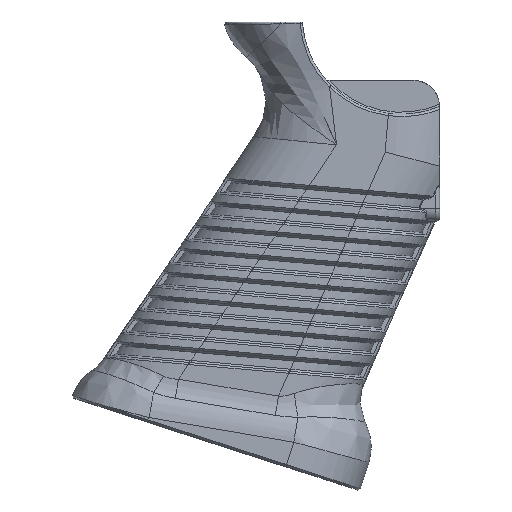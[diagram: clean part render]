
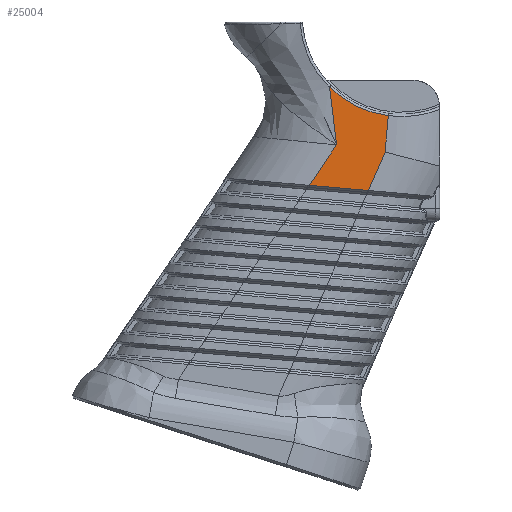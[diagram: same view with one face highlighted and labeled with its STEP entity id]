
A CAD part, top view. The second image highlights one B-rep face of the part: STEP entity #25004.
In plain terms, the highlighted planar face has unit normal (0, 0, 1).
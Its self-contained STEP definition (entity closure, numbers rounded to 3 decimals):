
#43 = DIRECTION ( 'NONE',  ( 0., 0., -1. ) ) ;
#418 = ORIENTED_EDGE ( 'NONE', *, *, #11434, .F. ) ;
#522 = DIRECTION ( 'NONE',  ( 0., 0., 1. ) ) ;
#1419 = VECTOR ( 'NONE', #10478, 1000. ) ;
#3633 = CARTESIAN_POINT ( 'NONE',  ( -142.328, -35.946, 17.501 ) ) ;
#3802 = VECTOR ( 'NONE', #4285, 1000. ) ;
#4087 = LINE ( 'NONE', #6663, #24403 ) ;
#4285 = DIRECTION ( 'NONE',  ( -0.996, 0.087, 0. ) ) ;
#4435 = VERTEX_POINT ( 'NONE', #27079 ) ;
#4528 = VERTEX_POINT ( 'NONE', #9547 ) ;
#5375 = EDGE_CURVE ( 'NONE', #19435, #14059, #4087, .T. ) ;
#5696 = LINE ( 'NONE', #3633, #17031 ) ;
#5759 = EDGE_CURVE ( 'NONE', #14059, #4528, #22493, .T. ) ;
#5824 = CARTESIAN_POINT ( 'NONE',  ( -158.322, -37.684, 17.501 ) ) ;
#6024 = CARTESIAN_POINT ( 'NONE',  ( -159.225, -30.876, 17.501 ) ) ;
#6251 = CARTESIAN_POINT ( 'NONE',  ( -158.847, -33.206, 17.501 ) ) ;
#6663 = CARTESIAN_POINT ( 'NONE',  ( -146.326, -26.223, 17.501 ) ) ;
#7158 = ORIENTED_EDGE ( 'NONE', *, *, #5759, .F. ) ;
#7208 = CARTESIAN_POINT ( 'NONE',  ( -132.232, -35.729, 17.501 ) ) ;
#7649 = FACE_OUTER_BOUND ( 'NONE', #9643, .T. ) ;
#7962 = CARTESIAN_POINT ( 'NONE',  ( -164.336, -52.925, 17.501 ) ) ;
#8347 = CARTESIAN_POINT ( 'NONE',  ( -159.467, -29.661, 17.501 ) ) ;
#9547 = CARTESIAN_POINT ( 'NONE',  ( -159.489, -29.553, 17.501 ) ) ;
#9643 = EDGE_LOOP ( 'NONE', ( #418, #7158, #22928, #22411, #29235, #12573, #22606 ) ) ;
#9734 = CARTESIAN_POINT ( 'NONE',  ( -145.543, -36.362, 17.501 ) ) ;
#9967 = DIRECTION ( 'NONE',  ( -0.559, -0.829, 0. ) ) ;
#10478 = DIRECTION ( 'NONE',  ( -0.996, 0.087, 0. ) ) ;
#10980 = CARTESIAN_POINT ( 'NONE',  ( -158.047, -41.059, 17.501 ) ) ;
#11176 = CARTESIAN_POINT ( 'NONE',  ( -157.86, -43.311, 17.501 ) ) ;
#11434 = EDGE_CURVE ( 'NONE', #4528, #17781, #12919, .T. ) ;
#11698 = LINE ( 'NONE', #31031, #32031 ) ;
#12573 = ORIENTED_EDGE ( 'NONE', *, *, #16999, .T. ) ;
#12758 = DIRECTION ( 'NONE',  ( -0.454, -0.891, 0. ) ) ;
#12919 = CIRCLE ( 'NONE', #29790, 24. ) ;
#13386 = CARTESIAN_POINT ( 'NONE',  ( -159.489, -29.553, 17.501 ) ) ;
#13405 = EDGE_CURVE ( 'NONE', #15309, #19435, #20616, .T. ) ;
#13424 = CARTESIAN_POINT ( 'NONE',  ( -157.859, -43.322, 17.501 ) ) ;
#14059 = VERTEX_POINT ( 'NONE', #13424 ) ;
#14193 = AXIS2_PLACEMENT_3D ( 'NONE', #7208, #43, #9967 ) ;
#14888 = PLANE ( 'NONE',  #14193 ) ;
#15309 = VERTEX_POINT ( 'NONE', #19824 ) ;
#16999 = EDGE_CURVE ( 'NONE', #31300, #4435, #5696, .T. ) ;
#17031 = VECTOR ( 'NONE', #31422, 1000. ) ;
#17781 = VERTEX_POINT ( 'NONE', #9734 ) ;
#17807 = CARTESIAN_POINT ( 'NONE',  ( -150.283, -54.154, 17.501 ) ) ;
#18905 = DIRECTION ( 'NONE',  ( 0.559, 0.829, 0. ) ) ;
#19435 = VERTEX_POINT ( 'NONE', #7962 ) ;
#19618 = CARTESIAN_POINT ( 'NONE',  ( -150.283, -54.154, 17.501 ) ) ;
#19824 = CARTESIAN_POINT ( 'NONE',  ( -150.45, -54.139, 17.501 ) ) ;
#20478 = CARTESIAN_POINT ( 'NONE',  ( -142.551, -12.55, 17.501 ) ) ;
#20616 = LINE ( 'NONE', #23982, #3802 ) ;
#20953 = LINE ( 'NONE', #17807, #1419 ) ;
#20997 = CARTESIAN_POINT ( 'NONE',  ( -157.859, -43.322, 17.501 ) ) ;
#21176 = EDGE_CURVE ( 'NONE', #17781, #4435, #11698, .T. ) ;
#22411 = ORIENTED_EDGE ( 'NONE', *, *, #13405, .F. ) ;
#22493 = B_SPLINE_CURVE_WITH_KNOTS ( 'NONE', 3,
 ( #20997, #23650, #11176, #10980, #5824, #6251, #6024, #8347, #13386 ),
 .UNSPECIFIED., .F., .F.,
 ( 4, 2, 1, 1, 1, 4 ),
 ( -0.002, 0., 0.676, 1.014, 1.352, 1.385 ),
 .UNSPECIFIED. ) ;
#22606 = ORIENTED_EDGE ( 'NONE', *, *, #21176, .F. ) ;
#22928 = ORIENTED_EDGE ( 'NONE', *, *, #5375, .F. ) ;
#23375 = DIRECTION ( 'NONE',  ( -0.087, -0.996, 0. ) ) ;
#23650 = CARTESIAN_POINT ( 'NONE',  ( -157.86, -43.317, 17.501 ) ) ;
#23982 = CARTESIAN_POINT ( 'NONE',  ( -143.754, -54.725, 17.501 ) ) ;
#24339 = EDGE_CURVE ( 'NONE', #31300, #15309, #20953, .T. ) ;
#24403 = VECTOR ( 'NONE', #18905, 1000. ) ;
#25004 = ADVANCED_FACE ( 'NONE', ( #7649 ), #14888, .F. ) ;
#27079 = CARTESIAN_POINT ( 'NONE',  ( -146.303, -45.044, 17.501 ) ) ;
#29235 = ORIENTED_EDGE ( 'NONE', *, *, #24339, .F. ) ;
#29790 = AXIS2_PLACEMENT_3D ( 'NONE', #20478, #522, #12758 ) ;
#31031 = CARTESIAN_POINT ( 'NONE',  ( -145.879, -40.205, 17.501 ) ) ;
#31300 = VERTEX_POINT ( 'NONE', #19618 ) ;
#31422 = DIRECTION ( 'NONE',  ( 0.4, 0.916, 0. ) ) ;
#32031 = VECTOR ( 'NONE', #23375, 1000. ) ;
